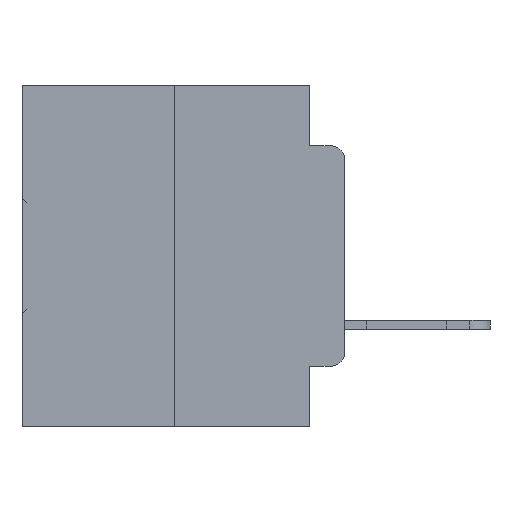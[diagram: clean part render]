
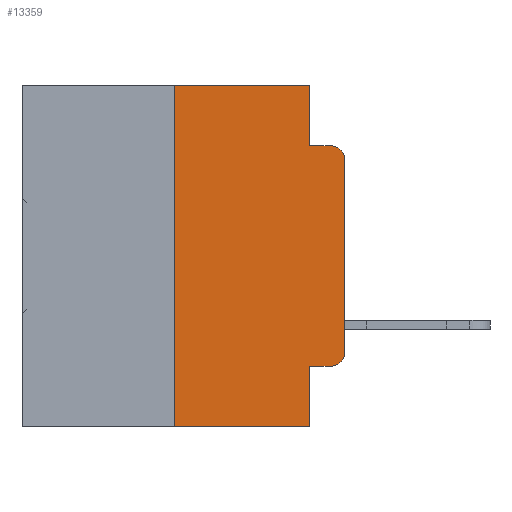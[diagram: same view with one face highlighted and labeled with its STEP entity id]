
A CAD part, left-side view. The second image highlights one B-rep face of the part: STEP entity #13359.
In plain terms, the highlighted planar face has unit normal (-1, 0, 0).
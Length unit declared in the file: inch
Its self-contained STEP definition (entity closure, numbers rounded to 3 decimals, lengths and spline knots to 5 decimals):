
#311 = VECTOR ( 'NONE', #3604, 39.37008 ) ;
#551 = CARTESIAN_POINT ( 'NONE',  ( 0., 0.473, -0.5 ) ) ;
#686 = VERTEX_POINT ( 'NONE', #13842 ) ;
#1384 = VECTOR ( 'NONE', #16690, 39.37008 ) ;
#1446 = EDGE_LOOP ( 'NONE', ( #6136, #6200, #6713, #6748, #7169, #7305, #7667, #7739, #8156, #8226 ) ) ;
#1531 = CARTESIAN_POINT ( 'NONE',  ( 0., 0.051, 0. ) ) ;
#1552 = EDGE_CURVE ( 'NONE', #33185, #23759, #7938, .T. ) ;
#1885 = VERTEX_POINT ( 'NONE', #34203 ) ;
#2437 = CARTESIAN_POINT ( 'NONE',  ( 0., 0.473, 0. ) ) ;
#3474 = DIRECTION ( 'NONE',  ( 0., -1., 0. ) ) ;
#3604 = DIRECTION ( 'NONE',  ( 0., -1., 0. ) ) ;
#4350 = DIRECTION ( 'NONE',  ( 0., 0., 1. ) ) ;
#4683 = LINE ( 'NONE', #24411, #32326 ) ;
#5239 = DIRECTION ( 'NONE',  ( 0., -1., 0. ) ) ;
#5576 = LINE ( 'NONE', #27329, #12231 ) ;
#6136 = ORIENTED_EDGE ( 'NONE', *, *, #12332, .T. ) ;
#6200 = ORIENTED_EDGE ( 'NONE', *, *, #12294, .T. ) ;
#6713 = ORIENTED_EDGE ( 'NONE', *, *, #12856, .F. ) ;
#6748 = ORIENTED_EDGE ( 'NONE', *, *, #25927, .F. ) ;
#6873 = CARTESIAN_POINT ( 'NONE',  ( 0., 0., -0.1085 ) ) ;
#6895 = CARTESIAN_POINT ( 'NONE',  ( 0., 0.473, 0. ) ) ;
#7169 = ORIENTED_EDGE ( 'NONE', *, *, #1552, .F. ) ;
#7305 = ORIENTED_EDGE ( 'NONE', *, *, #17990, .F. ) ;
#7667 = ORIENTED_EDGE ( 'NONE', *, *, #13016, .T. ) ;
#7739 = ORIENTED_EDGE ( 'NONE', *, *, #23564, .F. ) ;
#7938 = LINE ( 'NONE', #6895, #311 ) ;
#8156 = ORIENTED_EDGE ( 'NONE', *, *, #33043, .T. ) ;
#8159 = DIRECTION ( 'NONE',  ( 1., 0., 0. ) ) ;
#8226 = ORIENTED_EDGE ( 'NONE', *, *, #32281, .T. ) ;
#8246 = CARTESIAN_POINT ( 'NONE',  ( 0., 0.02, -0.0885 ) ) ;
#8276 = VERTEX_POINT ( 'NONE', #26982 ) ;
#8573 = DIRECTION ( 'NONE',  ( 0., 0., 1. ) ) ;
#8780 = FACE_OUTER_BOUND ( 'NONE', #1446, .T. ) ;
#11139 = CARTESIAN_POINT ( 'NONE',  ( 0., 0.051, 0. ) ) ;
#11309 = CARTESIAN_POINT ( 'NONE',  ( 0., 0.02, -0.1085 ) ) ;
#12231 = VECTOR ( 'NONE', #8573, 39.37008 ) ;
#12294 = EDGE_CURVE ( 'NONE', #12555, #19075, #21129, .T. ) ;
#12332 = EDGE_CURVE ( 'NONE', #8276, #12555, #5576, .T. ) ;
#12555 = VERTEX_POINT ( 'NONE', #6873 ) ;
#12856 = EDGE_CURVE ( 'NONE', #686, #19075, #4683, .T. ) ;
#13016 = EDGE_CURVE ( 'NONE', #19630, #1885, #32723, .T. ) ;
#13359 = ADVANCED_FACE ( 'NONE', ( #8780 ), #21701, .F. ) ;
#13523 = LINE ( 'NONE', #1531, #19924 ) ;
#13524 = AXIS2_PLACEMENT_3D ( 'NONE', #2437, #8159, #26959 ) ;
#13842 = CARTESIAN_POINT ( 'NONE',  ( 0., 0.051, -0.0885 ) ) ;
#13898 = AXIS2_PLACEMENT_3D ( 'NONE', #16543, #34558, #19263 ) ;
#14100 = DIRECTION ( 'NONE',  ( 0., 0., -1. ) ) ;
#15836 = VECTOR ( 'NONE', #5239, 39.37008 ) ;
#16543 = CARTESIAN_POINT ( 'NONE',  ( 0., 0.02, -0.3915 ) ) ;
#16690 = DIRECTION ( 'NONE',  ( 0., 0., -1. ) ) ;
#17266 = VERTEX_POINT ( 'NONE', #31889 ) ;
#17990 = EDGE_CURVE ( 'NONE', #19630, #33185, #30922, .T. ) ;
#18026 = VECTOR ( 'NONE', #4350, 39.37008 ) ;
#18400 = CARTESIAN_POINT ( 'NONE',  ( 0., 0.25, 0. ) ) ;
#19059 = VECTOR ( 'NONE', #3474, 39.37008 ) ;
#19075 = VERTEX_POINT ( 'NONE', #8246 ) ;
#19263 = DIRECTION ( 'NONE',  ( 0., 0., -1. ) ) ;
#19346 = DIRECTION ( 'NONE',  ( 0., -1., 0. ) ) ;
#19630 = VERTEX_POINT ( 'NONE', #29012 ) ;
#19924 = VECTOR ( 'NONE', #21009, 39.37008 ) ;
#21009 = DIRECTION ( 'NONE',  ( 0., 0., -1. ) ) ;
#21129 = CIRCLE ( 'NONE', #30188, 0.02 ) ;
#21701 = PLANE ( 'NONE',  #13524 ) ;
#23564 = EDGE_CURVE ( 'NONE', #17266, #1885, #13523, .T. ) ;
#23759 = VERTEX_POINT ( 'NONE', #26835 ) ;
#24411 = CARTESIAN_POINT ( 'NONE',  ( 0., 0.051, -0.0885 ) ) ;
#24848 = CARTESIAN_POINT ( 'NONE',  ( 0., 0.25, 0. ) ) ;
#25927 = EDGE_CURVE ( 'NONE', #23759, #686, #30195, .T. ) ;
#26835 = CARTESIAN_POINT ( 'NONE',  ( 0., 0.051, 0. ) ) ;
#26895 = VERTEX_POINT ( 'NONE', #33371 ) ;
#26959 = DIRECTION ( 'NONE',  ( 0., 0., -1. ) ) ;
#26982 = CARTESIAN_POINT ( 'NONE',  ( 0., 0., -0.3915 ) ) ;
#27329 = CARTESIAN_POINT ( 'NONE',  ( 0., 0., 0. ) ) ;
#29012 = CARTESIAN_POINT ( 'NONE',  ( 0., 0.25, -0.5 ) ) ;
#29437 = CARTESIAN_POINT ( 'NONE',  ( 0., 0.051, -0.4115 ) ) ;
#29662 = LINE ( 'NONE', #29437, #15836 ) ;
#29769 = DIRECTION ( 'NONE',  ( -1., 0., 0. ) ) ;
#30188 = AXIS2_PLACEMENT_3D ( 'NONE', #11309, #29769, #14100 ) ;
#30195 = LINE ( 'NONE', #11139, #1384 ) ;
#30922 = LINE ( 'NONE', #18400, #18026 ) ;
#31889 = CARTESIAN_POINT ( 'NONE',  ( 0., 0.051, -0.4115 ) ) ;
#32281 = EDGE_CURVE ( 'NONE', #26895, #8276, #34434, .T. ) ;
#32326 = VECTOR ( 'NONE', #19346, 39.37008 ) ;
#32723 = LINE ( 'NONE', #551, #19059 ) ;
#33043 = EDGE_CURVE ( 'NONE', #17266, #26895, #29662, .T. ) ;
#33185 = VERTEX_POINT ( 'NONE', #24848 ) ;
#33371 = CARTESIAN_POINT ( 'NONE',  ( 0., 0.02, -0.4115 ) ) ;
#34203 = CARTESIAN_POINT ( 'NONE',  ( 0., 0.051, -0.5 ) ) ;
#34434 = CIRCLE ( 'NONE', #13898, 0.02 ) ;
#34558 = DIRECTION ( 'NONE',  ( -1., 0., 0. ) ) ;
